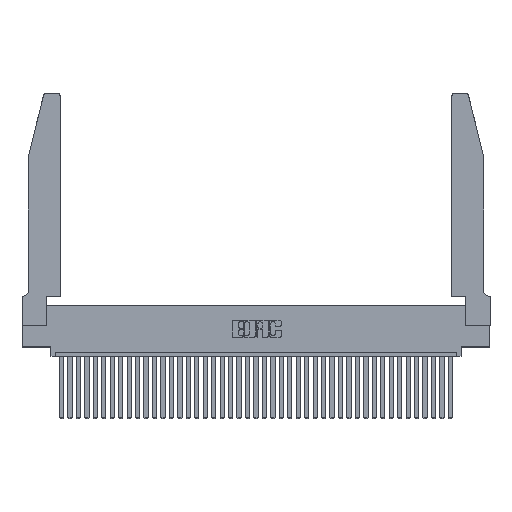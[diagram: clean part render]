
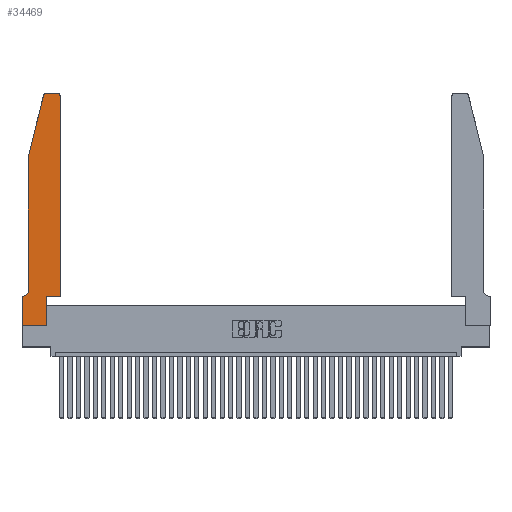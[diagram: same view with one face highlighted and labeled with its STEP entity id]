
A CAD part, top view. The second image highlights one B-rep face of the part: STEP entity #34469.
In plain terms, the highlighted planar face has unit normal (0, 0, 1).
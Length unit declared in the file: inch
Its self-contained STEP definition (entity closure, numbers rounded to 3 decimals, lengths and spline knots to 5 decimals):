
#57 = EDGE_CURVE ( 'NONE', #26038, #21673, #15233, .T. ) ;
#1104 = VERTEX_POINT ( 'NONE', #7077 ) ;
#1180 = CIRCLE ( 'NONE', #28866, 0.03 ) ;
#1262 = DIRECTION ( 'NONE',  ( 0., -1., 0. ) ) ;
#1455 = CARTESIAN_POINT ( 'NONE',  ( 0.4205, 2.72, 0.37 ) ) ;
#1709 = DIRECTION ( 'NONE',  ( 0., 0., 1. ) ) ;
#1973 = PLANE ( 'NONE',  #14775 ) ;
#2046 = CARTESIAN_POINT ( 'NONE',  ( 0.4505, 0.35, 0.37 ) ) ;
#2090 = DIRECTION ( 'NONE',  ( 1., 0., 0. ) ) ;
#2560 = CARTESIAN_POINT ( 'NONE',  ( 0.2865, 0., 0.37 ) ) ;
#2790 = DIRECTION ( 'NONE',  ( -1., 0., 0. ) ) ;
#3307 = EDGE_CURVE ( 'NONE', #16903, #8885, #14928, .T. ) ;
#3822 = CARTESIAN_POINT ( 'NONE',  ( 0., 0.35, 0.37 ) ) ;
#3901 = VECTOR ( 'NONE', #1262, 39.37008 ) ;
#4652 = CARTESIAN_POINT ( 'NONE',  ( 0., 0.35, 0.37 ) ) ;
#4814 = VERTEX_POINT ( 'NONE', #2046 ) ;
#7077 = CARTESIAN_POINT ( 'NONE',  ( 0.0755, 0.42, 0.37 ) ) ;
#7133 = VECTOR ( 'NONE', #22871, 39.37008 ) ;
#7773 = LINE ( 'NONE', #30028, #19162 ) ;
#8437 = VERTEX_POINT ( 'NONE', #37064 ) ;
#8885 = VERTEX_POINT ( 'NONE', #3822 ) ;
#9035 = CARTESIAN_POINT ( 'NONE',  ( 0.4505, 0.35, 0.37 ) ) ;
#9460 = CARTESIAN_POINT ( 'NONE',  ( 0.284, 2.75, 0.37 ) ) ;
#10236 = VECTOR ( 'NONE', #29300, 39.37008 ) ;
#10346 = ORIENTED_EDGE ( 'NONE', *, *, #19701, .T. ) ;
#10487 = ORIENTED_EDGE ( 'NONE', *, *, #24402, .T. ) ;
#10616 = CARTESIAN_POINT ( 'NONE',  ( 0., 0., 0.37 ) ) ;
#10695 = VECTOR ( 'NONE', #22593, 39.37008 ) ;
#10958 = CARTESIAN_POINT ( 'NONE',  ( 0.0755, 2., 0.37 ) ) ;
#11626 = ORIENTED_EDGE ( 'NONE', *, *, #57, .T. ) ;
#11843 = VERTEX_POINT ( 'NONE', #33186 ) ;
#13387 = EDGE_CURVE ( 'NONE', #11843, #1104, #15405, .T. ) ;
#14003 = EDGE_CURVE ( 'NONE', #8885, #32794, #30539, .T. ) ;
#14581 = AXIS2_PLACEMENT_3D ( 'NONE', #15012, #21007, #2790 ) ;
#14698 = EDGE_LOOP ( 'NONE', ( #15581, #10487, #10346, #18844, #27530, #24586, #23917, #20313, #11626, #19812, #26777, #18668 ) ) ;
#14775 = AXIS2_PLACEMENT_3D ( 'NONE', #4652, #1709, #29124 ) ;
#14801 = DIRECTION ( 'NONE',  ( 0., 0., 1. ) ) ;
#14928 = LINE ( 'NONE', #15477, #20661 ) ;
#15012 = CARTESIAN_POINT ( 'NONE',  ( 0.0055, 0.42, 0.37 ) ) ;
#15233 = LINE ( 'NONE', #29521, #7133 ) ;
#15382 = CIRCLE ( 'NONE', #35401, 0.03 ) ;
#15405 = LINE ( 'NONE', #38761, #10236 ) ;
#15477 = CARTESIAN_POINT ( 'NONE',  ( 0.0755, 0.35, 0.37 ) ) ;
#15581 = ORIENTED_EDGE ( 'NONE', *, *, #18703, .T. ) ;
#16611 = CARTESIAN_POINT ( 'NONE',  ( 0.2605, 2.75, 0.37 ) ) ;
#16903 = VERTEX_POINT ( 'NONE', #26708 ) ;
#18668 = ORIENTED_EDGE ( 'NONE', *, *, #18854, .T. ) ;
#18703 = EDGE_CURVE ( 'NONE', #8437, #29057, #19705, .T. ) ;
#18844 = ORIENTED_EDGE ( 'NONE', *, *, #13387, .T. ) ;
#18854 = EDGE_CURVE ( 'NONE', #25901, #8437, #15382, .T. ) ;
#18912 = VECTOR ( 'NONE', #30058, 39.37008 ) ;
#19057 = CARTESIAN_POINT ( 'NONE',  ( 0., 0., 0.37 ) ) ;
#19162 = VECTOR ( 'NONE', #2090, 39.37008 ) ;
#19701 = EDGE_CURVE ( 'NONE', #24267, #11843, #26028, .T. ) ;
#19705 = LINE ( 'NONE', #16611, #10695 ) ;
#19812 = ORIENTED_EDGE ( 'NONE', *, *, #25171, .T. ) ;
#20313 = ORIENTED_EDGE ( 'NONE', *, *, #34384, .T. ) ;
#20661 = VECTOR ( 'NONE', #22130, 39.37008 ) ;
#21007 = DIRECTION ( 'NONE',  ( 0., 0., -1. ) ) ;
#21276 = CIRCLE ( 'NONE', #14581, 0.07 ) ;
#21673 = VERTEX_POINT ( 'NONE', #29546 ) ;
#22130 = DIRECTION ( 'NONE',  ( -1., 0., 0. ) ) ;
#22593 = DIRECTION ( 'NONE',  ( -1., 0., 0. ) ) ;
#22871 = DIRECTION ( 'NONE',  ( 0., 1., 0. ) ) ;
#23538 = EDGE_CURVE ( 'NONE', #1104, #16903, #21276, .T. ) ;
#23917 = ORIENTED_EDGE ( 'NONE', *, *, #14003, .T. ) ;
#24003 = LINE ( 'NONE', #34180, #27817 ) ;
#24267 = VERTEX_POINT ( 'NONE', #25202 ) ;
#24402 = EDGE_CURVE ( 'NONE', #29057, #24267, #1180, .T. ) ;
#24586 = ORIENTED_EDGE ( 'NONE', *, *, #3307, .T. ) ;
#25171 = EDGE_CURVE ( 'NONE', #21673, #4814, #7773, .T. ) ;
#25202 = CARTESIAN_POINT ( 'NONE',  ( 0.25487, 2.72718, 0.37 ) ) ;
#25901 = VERTEX_POINT ( 'NONE', #28662 ) ;
#25971 = CARTESIAN_POINT ( 'NONE',  ( 0.284, 2.72, 0.37 ) ) ;
#26028 = LINE ( 'NONE', #10958, #36519 ) ;
#26038 = VERTEX_POINT ( 'NONE', #2560 ) ;
#26367 = DIRECTION ( 'NONE',  ( 1., 0., 0. ) ) ;
#26390 = FACE_OUTER_BOUND ( 'NONE', #14698, .T. ) ;
#26708 = CARTESIAN_POINT ( 'NONE',  ( 0.0055, 0.35, 0.37 ) ) ;
#26777 = ORIENTED_EDGE ( 'NONE', *, *, #38834, .T. ) ;
#27522 = LINE ( 'NONE', #9035, #18912 ) ;
#27530 = ORIENTED_EDGE ( 'NONE', *, *, #23538, .T. ) ;
#27817 = VECTOR ( 'NONE', #28602, 39.37008 ) ;
#28602 = DIRECTION ( 'NONE',  ( 1., 0., 0. ) ) ;
#28662 = CARTESIAN_POINT ( 'NONE',  ( 0.4505, 2.72, 0.37 ) ) ;
#28866 = AXIS2_PLACEMENT_3D ( 'NONE', #25971, #32130, #26367 ) ;
#29057 = VERTEX_POINT ( 'NONE', #9460 ) ;
#29124 = DIRECTION ( 'NONE',  ( 1., 0., 0. ) ) ;
#29300 = DIRECTION ( 'NONE',  ( 0., -1., 0. ) ) ;
#29521 = CARTESIAN_POINT ( 'NONE',  ( 0.2865, 0.35, 0.37 ) ) ;
#29546 = CARTESIAN_POINT ( 'NONE',  ( 0.2865, 0.35, 0.37 ) ) ;
#30028 = CARTESIAN_POINT ( 'NONE',  ( 0.4505, 0.35, 0.37 ) ) ;
#30058 = DIRECTION ( 'NONE',  ( 0., 1., 0. ) ) ;
#30539 = LINE ( 'NONE', #10616, #3901 ) ;
#31203 = DIRECTION ( 'NONE',  ( 1., 0., 0. ) ) ;
#32130 = DIRECTION ( 'NONE',  ( 0., 0., 1. ) ) ;
#32794 = VERTEX_POINT ( 'NONE', #19057 ) ;
#33011 = DIRECTION ( 'NONE',  ( -0.239, -0.971, 0. ) ) ;
#33186 = CARTESIAN_POINT ( 'NONE',  ( 0.0755, 2., 0.37 ) ) ;
#34180 = CARTESIAN_POINT ( 'NONE',  ( 0., 0., 0.37 ) ) ;
#34384 = EDGE_CURVE ( 'NONE', #32794, #26038, #24003, .T. ) ;
#34469 = ADVANCED_FACE ( 'NONE', ( #26390 ), #1973, .T. ) ;
#35401 = AXIS2_PLACEMENT_3D ( 'NONE', #1455, #14801, #31203 ) ;
#36519 = VECTOR ( 'NONE', #33011, 39.37008 ) ;
#37064 = CARTESIAN_POINT ( 'NONE',  ( 0.4205, 2.75, 0.37 ) ) ;
#38761 = CARTESIAN_POINT ( 'NONE',  ( 0.0755, 2., 0.37 ) ) ;
#38834 = EDGE_CURVE ( 'NONE', #4814, #25901, #27522, .T. ) ;
